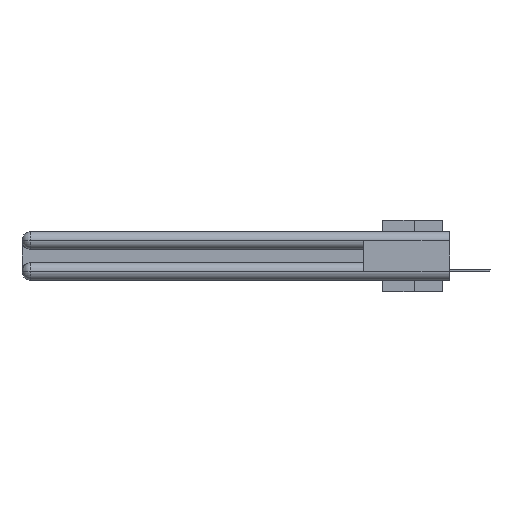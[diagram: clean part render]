
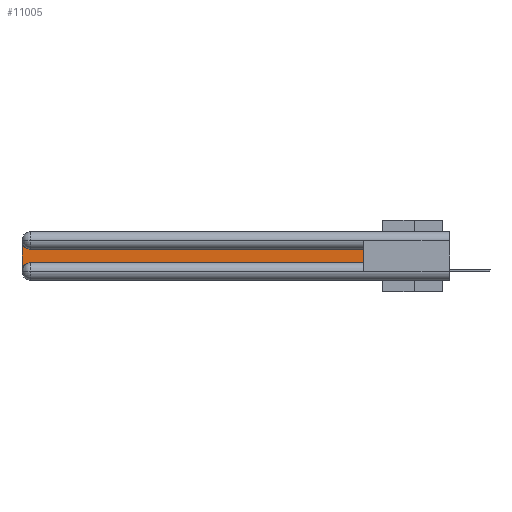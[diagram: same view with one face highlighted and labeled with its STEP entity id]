
A CAD part, left-side view. The second image highlights one B-rep face of the part: STEP entity #11005.
In plain terms, the highlighted planar face has unit normal (-1, 0, 0).
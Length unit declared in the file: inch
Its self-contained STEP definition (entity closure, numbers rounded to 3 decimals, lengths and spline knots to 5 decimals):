
#604 = CARTESIAN_POINT ( 'NONE',  ( 0.075, 2.94, -0.1225 ) ) ;
#1439 = DIRECTION ( 'NONE',  ( 0., 0., 1. ) ) ;
#1682 = DIRECTION ( 'NONE',  ( 0., 1., 0. ) ) ;
#1863 = VERTEX_POINT ( 'NONE', #14037 ) ;
#2277 = VERTEX_POINT ( 'NONE', #11515 ) ;
#2866 = LINE ( 'NONE', #30560, #23967 ) ;
#4404 = CARTESIAN_POINT ( 'NONE',  ( 0.075, 3., -0.2775 ) ) ;
#4504 = AXIS2_PLACEMENT_3D ( 'NONE', #26483, #12323, #29771 ) ;
#4525 = DIRECTION ( 'NONE',  ( 0., 0., -1. ) ) ;
#6881 = ORIENTED_EDGE ( 'NONE', *, *, #7423, .T. ) ;
#6994 = ORIENTED_EDGE ( 'NONE', *, *, #25591, .T. ) ;
#7058 = EDGE_LOOP ( 'NONE', ( #23057, #25600, #6881, #19802, #11149, #6994 ) ) ;
#7138 = LINE ( 'NONE', #17236, #8169 ) ;
#7423 = EDGE_CURVE ( 'NONE', #2277, #29229, #2866, .T. ) ;
#8169 = VECTOR ( 'NONE', #1682, 39.37008 ) ;
#8715 = DIRECTION ( 'NONE',  ( 1., 0., 0. ) ) ;
#9773 = VECTOR ( 'NONE', #22858, 39.37008 ) ;
#9994 = AXIS2_PLACEMENT_3D ( 'NONE', #11198, #8715, #4525 ) ;
#11005 = ADVANCED_FACE ( 'NONE', ( #12540 ), #22966, .F. ) ;
#11149 = ORIENTED_EDGE ( 'NONE', *, *, #29649, .T. ) ;
#11198 = CARTESIAN_POINT ( 'NONE',  ( 0.075, 2.94, -0.2775 ) ) ;
#11353 = CARTESIAN_POINT ( 'NONE',  ( 0.075, 0.6, -0.2175 ) ) ;
#11515 = CARTESIAN_POINT ( 'NONE',  ( 0.075, 3., -0.0625 ) ) ;
#12323 = DIRECTION ( 'NONE',  ( 1., 0., 0. ) ) ;
#12540 = FACE_OUTER_BOUND ( 'NONE', #7058, .T. ) ;
#12598 = LINE ( 'NONE', #27366, #9773 ) ;
#13831 = VECTOR ( 'NONE', #1439, 39.37008 ) ;
#14037 = CARTESIAN_POINT ( 'NONE',  ( 0.075, 0.6, -0.2175 ) ) ;
#14930 = EDGE_CURVE ( 'NONE', #29229, #21404, #30128, .T. ) ;
#15177 = CARTESIAN_POINT ( 'NONE',  ( 0.075, 2.94, -0.2175 ) ) ;
#16122 = CIRCLE ( 'NONE', #4504, 0.06 ) ;
#16824 = LINE ( 'NONE', #11353, #13831 ) ;
#17236 = CARTESIAN_POINT ( 'NONE',  ( 0.075, 0.6, -0.1225 ) ) ;
#19802 = ORIENTED_EDGE ( 'NONE', *, *, #14930, .T. ) ;
#20331 = VERTEX_POINT ( 'NONE', #604 ) ;
#21404 = VERTEX_POINT ( 'NONE', #15177 ) ;
#22805 = CARTESIAN_POINT ( 'NONE',  ( 0.075, 3., -0.1225 ) ) ;
#22858 = DIRECTION ( 'NONE',  ( 0., -1., 0. ) ) ;
#22966 = PLANE ( 'NONE',  #23065 ) ;
#23057 = ORIENTED_EDGE ( 'NONE', *, *, #31247, .T. ) ;
#23065 = AXIS2_PLACEMENT_3D ( 'NONE', #22805, #26241, #27630 ) ;
#23967 = VECTOR ( 'NONE', #24606, 39.37008 ) ;
#24606 = DIRECTION ( 'NONE',  ( 0., 0., -1. ) ) ;
#25591 = EDGE_CURVE ( 'NONE', #1863, #30507, #16824, .T. ) ;
#25600 = ORIENTED_EDGE ( 'NONE', *, *, #31606, .T. ) ;
#26241 = DIRECTION ( 'NONE',  ( 1., 0., 0. ) ) ;
#26483 = CARTESIAN_POINT ( 'NONE',  ( 0.075, 2.94, -0.0625 ) ) ;
#27366 = CARTESIAN_POINT ( 'NONE',  ( 0.075, 0.6, -0.2175 ) ) ;
#27630 = DIRECTION ( 'NONE',  ( 0., 0., -1. ) ) ;
#29229 = VERTEX_POINT ( 'NONE', #4404 ) ;
#29649 = EDGE_CURVE ( 'NONE', #21404, #1863, #12598, .T. ) ;
#29771 = DIRECTION ( 'NONE',  ( 0., 0., -1. ) ) ;
#29946 = CARTESIAN_POINT ( 'NONE',  ( 0.075, 0.6, -0.1225 ) ) ;
#30128 = CIRCLE ( 'NONE', #9994, 0.06 ) ;
#30507 = VERTEX_POINT ( 'NONE', #29946 ) ;
#30560 = CARTESIAN_POINT ( 'NONE',  ( 0.075, 3., -0.2175 ) ) ;
#31247 = EDGE_CURVE ( 'NONE', #30507, #20331, #7138, .T. ) ;
#31606 = EDGE_CURVE ( 'NONE', #20331, #2277, #16122, .T. ) ;
